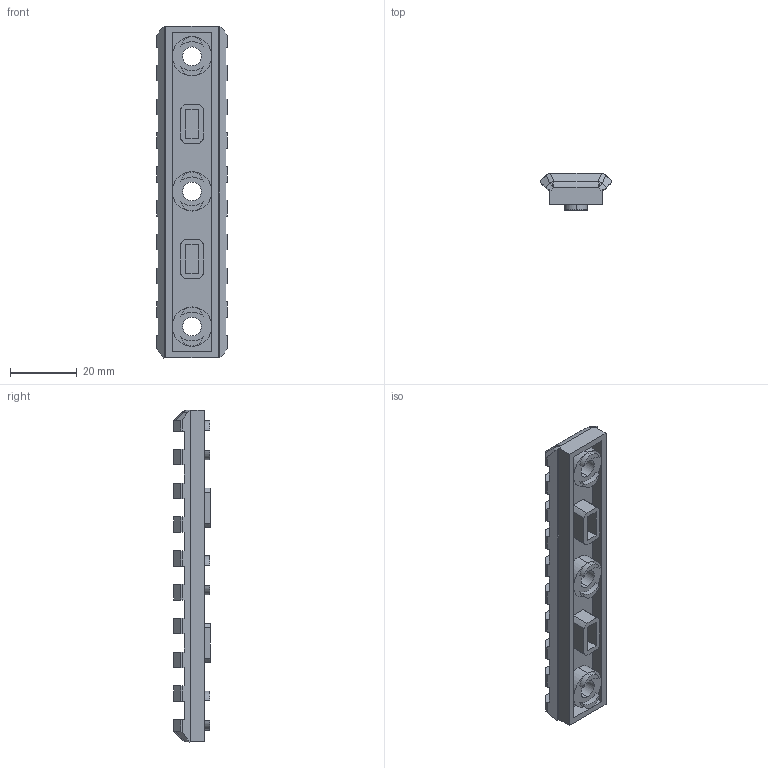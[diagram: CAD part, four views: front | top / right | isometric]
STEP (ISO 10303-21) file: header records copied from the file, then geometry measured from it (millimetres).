
FILE_DESCRIPTION (( 'STEP AP214' ), '1' );
FILE_NAME ('PICATINNY RAIL.step', '2019-12-18T03:08:22', ( '' ), ( '' ), 'SwSTEP 2.0', 'SolidWorks 2019', '' );
FILE_SCHEMA (( 'AUTOMOTIVE_DESIGN' ));
Length unit declared in the file: millimetre
Products named in the file (1): PICATINNY RAIL
Bounding box: 21.21 x 11.1 x 99.82 mm (x, y, z)
Volume: 9342.9 mm3; surface area: 9127.7 mm2
Topology: 1 solids, 1 shells, 209 faces, 567 edges, 374 vertices
Faces by surface type: plane 138, cylinder 36, bspline 35
Entity records: 9447 total; most frequent: CARTESIAN_POINT 4414, ORIENTED_EDGE 1134, DIRECTION 881, EDGE_CURVE 567, VERTEX_POINT 374, VECTOR 363, LINE 363, AXIS2_PLACEMENT_3D 259
